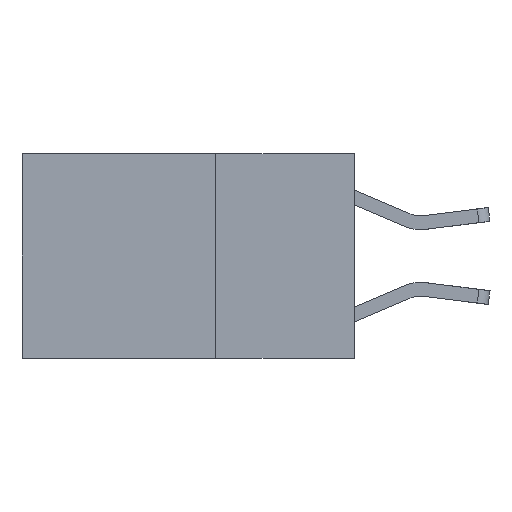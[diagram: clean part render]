
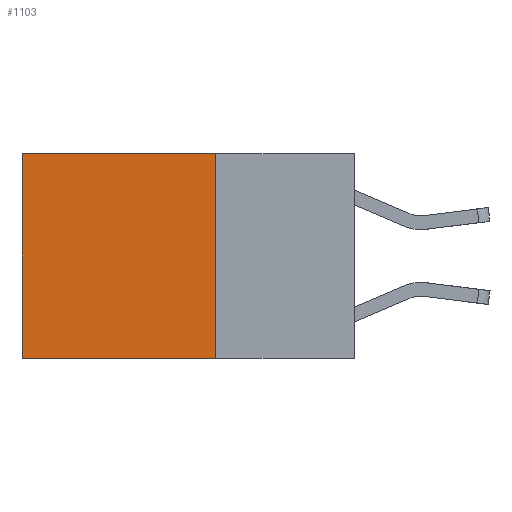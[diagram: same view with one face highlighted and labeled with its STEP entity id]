
A CAD part, left-side view. The second image highlights one B-rep face of the part: STEP entity #1103.
In plain terms, the highlighted planar face has unit normal (-1, 0, 0).
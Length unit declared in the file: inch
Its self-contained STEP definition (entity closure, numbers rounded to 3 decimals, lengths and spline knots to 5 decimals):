
#239 = DIRECTION ( 'NONE',  ( 1., 0., 0. ) ) ;
#395 = PLANE ( 'NONE',  #3487 ) ;
#492 = CARTESIAN_POINT ( 'NONE',  ( 0.2625, 0.25, 0. ) ) ;
#720 = FACE_OUTER_BOUND ( 'NONE', #3569, .T. ) ;
#1103 = ADVANCED_FACE ( 'NONE', ( #720 ), #395, .F. ) ;
#1107 = LINE ( 'NONE', #9067, #8576 ) ;
#1969 = VERTEX_POINT ( 'NONE', #2974 ) ;
#2210 = CARTESIAN_POINT ( 'NONE',  ( 0.2625, 0.25, 0. ) ) ;
#2443 = DIRECTION ( 'NONE',  ( 0., 0., -1. ) ) ;
#2783 = LINE ( 'NONE', #9574, #8290 ) ;
#2974 = CARTESIAN_POINT ( 'NONE',  ( 0.2625, 0.25, -0.37 ) ) ;
#3349 = DIRECTION ( 'NONE',  ( 0., 1., 0. ) ) ;
#3487 = AXIS2_PLACEMENT_3D ( 'NONE', #492, #239, #2443 ) ;
#3569 = EDGE_LOOP ( 'NONE', ( #6544, #4266, #4459, #4527 ) ) ;
#4266 = ORIENTED_EDGE ( 'NONE', *, *, #9783, .F. ) ;
#4459 = ORIENTED_EDGE ( 'NONE', *, *, #9040, .F. ) ;
#4514 = VECTOR ( 'NONE', #5971, 39.37008 ) ;
#4527 = ORIENTED_EDGE ( 'NONE', *, *, #5604, .T. ) ;
#5182 = LINE ( 'NONE', #8433, #8659 ) ;
#5367 = VERTEX_POINT ( 'NONE', #6757 ) ;
#5604 = EDGE_CURVE ( 'NONE', #7040, #5367, #5182, .T. ) ;
#5666 = DIRECTION ( 'NONE',  ( 0., 0., -1. ) ) ;
#5971 = DIRECTION ( 'NONE',  ( 0., 0., -1. ) ) ;
#6533 = LINE ( 'NONE', #2210, #4514 ) ;
#6544 = ORIENTED_EDGE ( 'NONE', *, *, #8866, .T. ) ;
#6757 = CARTESIAN_POINT ( 'NONE',  ( 0.2625, 0.6, 0. ) ) ;
#7040 = VERTEX_POINT ( 'NONE', #9157 ) ;
#7424 = VERTEX_POINT ( 'NONE', #8117 ) ;
#8117 = CARTESIAN_POINT ( 'NONE',  ( 0.2625, 0.6, -0.37 ) ) ;
#8136 = DIRECTION ( 'NONE',  ( 0., 1., 0. ) ) ;
#8290 = VECTOR ( 'NONE', #3349, 39.37008 ) ;
#8433 = CARTESIAN_POINT ( 'NONE',  ( 0.2625, 0.25, 0. ) ) ;
#8576 = VECTOR ( 'NONE', #5666, 39.37008 ) ;
#8659 = VECTOR ( 'NONE', #8136, 39.37008 ) ;
#8866 = EDGE_CURVE ( 'NONE', #5367, #7424, #1107, .T. ) ;
#9040 = EDGE_CURVE ( 'NONE', #7040, #1969, #6533, .T. ) ;
#9067 = CARTESIAN_POINT ( 'NONE',  ( 0.2625, 0.6, 0. ) ) ;
#9157 = CARTESIAN_POINT ( 'NONE',  ( 0.2625, 0.25, 0. ) ) ;
#9574 = CARTESIAN_POINT ( 'NONE',  ( 0.2625, 0.25, -0.37 ) ) ;
#9783 = EDGE_CURVE ( 'NONE', #1969, #7424, #2783, .T. ) ;
